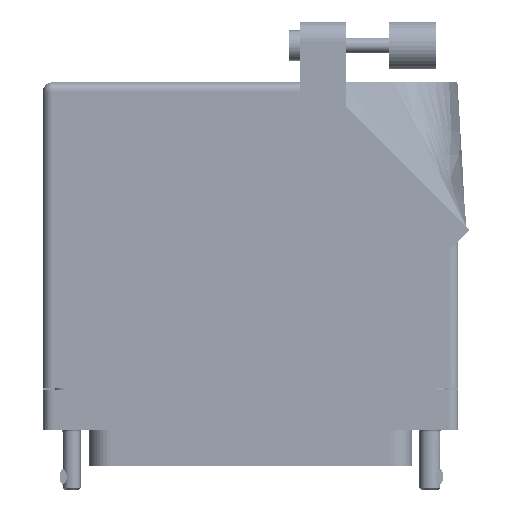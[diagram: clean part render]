
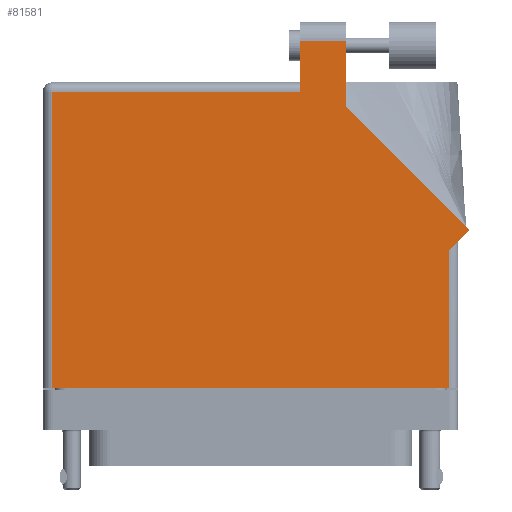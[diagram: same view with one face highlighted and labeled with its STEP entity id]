
A CAD part, front view. The second image highlights one B-rep face of the part: STEP entity #81581.
In plain terms, the highlighted face is planar.
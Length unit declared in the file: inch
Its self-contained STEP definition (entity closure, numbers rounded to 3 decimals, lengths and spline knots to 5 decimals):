
#758 = EDGE_CURVE ( 'NONE', #67585, #41093, #98569, .T. ) ;
#2305 = EDGE_CURVE ( 'NONE', #30783, #101381, #63682, .T. ) ;
#5697 = ORIENTED_EDGE ( 'NONE', *, *, #77650, .T. ) ;
#8278 = VERTEX_POINT ( 'NONE', #77160 ) ;
#10716 = CARTESIAN_POINT ( 'NONE',  ( -1.3775, 1.93, 0.765 ) ) ;
#10763 = VECTOR ( 'NONE', #30957, 39.37008 ) ;
#11295 = VECTOR ( 'NONE', #24238, 39.37008 ) ;
#14089 = EDGE_CURVE ( 'NONE', #31256, #15757, #40930, .T. ) ;
#15217 = CARTESIAN_POINT ( 'NONE',  ( 1.3775, 0.88, 0.765 ) ) ;
#15598 = CARTESIAN_POINT ( 'NONE',  ( -1.3155, 1.868, 0.765 ) ) ;
#15757 = VERTEX_POINT ( 'NONE', #60835 ) ;
#16546 = CARTESIAN_POINT ( 'NONE',  ( -1.3155, -0.1, 0.765 ) ) ;
#17217 = CARTESIAN_POINT ( 'NONE',  ( -1.3155, -0.1, 0.765 ) ) ;
#18351 = DIRECTION ( 'NONE',  ( -1., 0., 0. ) ) ;
#19984 = EDGE_CURVE ( 'NONE', #88259, #30783, #83841, .T. ) ;
#22496 = ORIENTED_EDGE ( 'NONE', *, *, #2305, .T. ) ;
#23642 = ORIENTED_EDGE ( 'NONE', *, *, #14089, .T. ) ;
#24238 = DIRECTION ( 'NONE',  ( 0., -1., 0. ) ) ;
#24266 = DIRECTION ( 'NONE',  ( 0.707, 0.707, 0. ) ) ;
#25860 = FACE_OUTER_BOUND ( 'NONE', #77735, .T. ) ;
#26349 = ORIENTED_EDGE ( 'NONE', *, *, #60284, .T. ) ;
#28736 = CARTESIAN_POINT ( 'NONE',  ( 0.3275, 2.205, 0.765 ) ) ;
#29810 = AXIS2_PLACEMENT_3D ( 'NONE', #10716, #97506, #18351 ) ;
#30783 = VERTEX_POINT ( 'NONE', #15598 ) ;
#30957 = DIRECTION ( 'NONE',  ( -0.707, 0.707, 0. ) ) ;
#30986 = VECTOR ( 'NONE', #64364, 39.37008 ) ;
#31256 = VERTEX_POINT ( 'NONE', #78378 ) ;
#32774 = VECTOR ( 'NONE', #85920, 39.37008 ) ;
#35843 = CARTESIAN_POINT ( 'NONE',  ( 0.3275, 1.868, 0.765 ) ) ;
#36242 = LINE ( 'NONE', #63251, #38712 ) ;
#38071 = CARTESIAN_POINT ( 'NONE',  ( 0.3275, 2.205, 0.765 ) ) ;
#38712 = VECTOR ( 'NONE', #71552, 39.37008 ) ;
#39484 = VECTOR ( 'NONE', #81829, 39.37008 ) ;
#40930 = LINE ( 'NONE', #72680, #30986 ) ;
#41093 = VERTEX_POINT ( 'NONE', #28736 ) ;
#41814 = CARTESIAN_POINT ( 'NONE',  ( 0.6345, 2.205, 0.765 ) ) ;
#43236 = LINE ( 'NONE', #65556, #39484 ) ;
#44797 = ORIENTED_EDGE ( 'NONE', *, *, #758, .T. ) ;
#55124 = EDGE_CURVE ( 'NONE', #41093, #88259, #43236, .T. ) ;
#57475 = VERTEX_POINT ( 'NONE', #80748 ) ;
#57624 = PLANE ( 'NONE',  #29810 ) ;
#60284 = EDGE_CURVE ( 'NONE', #101381, #31256, #88723, .T. ) ;
#60835 = CARTESIAN_POINT ( 'NONE',  ( 1.3155, 0.818, 0.765 ) ) ;
#63251 = CARTESIAN_POINT ( 'NONE',  ( 0.6345, 1.76442, 0.765 ) ) ;
#63682 = LINE ( 'NONE', #17217, #11295 ) ;
#64364 = DIRECTION ( 'NONE',  ( 0., 1., 0. ) ) ;
#65171 = VECTOR ( 'NONE', #73328, 39.37008 ) ;
#65556 = CARTESIAN_POINT ( 'NONE',  ( 0.3275, 1.93, 0.765 ) ) ;
#67585 = VERTEX_POINT ( 'NONE', #41814 ) ;
#68291 = ORIENTED_EDGE ( 'NONE', *, *, #79118, .T. ) ;
#69152 = EDGE_CURVE ( 'NONE', #8278, #57475, #100226, .T. ) ;
#71552 = DIRECTION ( 'NONE',  ( 0., 1., 0. ) ) ;
#72680 = CARTESIAN_POINT ( 'NONE',  ( 1.3155, 0.88, 0.765 ) ) ;
#72966 = CARTESIAN_POINT ( 'NONE',  ( -1.3775, -0.1, 0.765 ) ) ;
#73328 = DIRECTION ( 'NONE',  ( 1., 0., 0. ) ) ;
#77160 = CARTESIAN_POINT ( 'NONE',  ( 1.44821, 0.95071, 0.765 ) ) ;
#77321 = ORIENTED_EDGE ( 'NONE', *, *, #19984, .T. ) ;
#77650 = EDGE_CURVE ( 'NONE', #15757, #8278, #84519, .T. ) ;
#77735 = EDGE_LOOP ( 'NONE', ( #68291, #44797, #78757, #77321, #22496, #26349, #23642, #5697, #97227 ) ) ;
#78378 = CARTESIAN_POINT ( 'NONE',  ( 1.3155, -0.1, 0.765 ) ) ;
#78757 = ORIENTED_EDGE ( 'NONE', *, *, #55124, .T. ) ;
#79118 = EDGE_CURVE ( 'NONE', #57475, #67585, #36242, .T. ) ;
#80748 = CARTESIAN_POINT ( 'NONE',  ( 0.6345, 1.76442, 0.765 ) ) ;
#80842 = VECTOR ( 'NONE', #24266, 39.37008 ) ;
#81381 = VECTOR ( 'NONE', #87089, 39.37008 ) ;
#81581 = ADVANCED_FACE ( 'NONE', ( #25860 ), #57624, .F. ) ;
#81829 = DIRECTION ( 'NONE',  ( 0., -1., 0. ) ) ;
#83834 = CARTESIAN_POINT ( 'NONE',  ( -1.3775, 1.868, 0.765 ) ) ;
#83841 = LINE ( 'NONE', #83834, #81381 ) ;
#84519 = LINE ( 'NONE', #15217, #80842 ) ;
#85920 = DIRECTION ( 'NONE',  ( -1., 0., 0. ) ) ;
#86423 = CARTESIAN_POINT ( 'NONE',  ( 1.44821, 0.95071, 0.765 ) ) ;
#87089 = DIRECTION ( 'NONE',  ( -1., 0., 0. ) ) ;
#88259 = VERTEX_POINT ( 'NONE', #35843 ) ;
#88723 = LINE ( 'NONE', #72966, #65171 ) ;
#97227 = ORIENTED_EDGE ( 'NONE', *, *, #69152, .T. ) ;
#97506 = DIRECTION ( 'NONE',  ( 0., 0., -1. ) ) ;
#98569 = LINE ( 'NONE', #38071, #32774 ) ;
#100226 = LINE ( 'NONE', #86423, #10763 ) ;
#101381 = VERTEX_POINT ( 'NONE', #16546 ) ;
